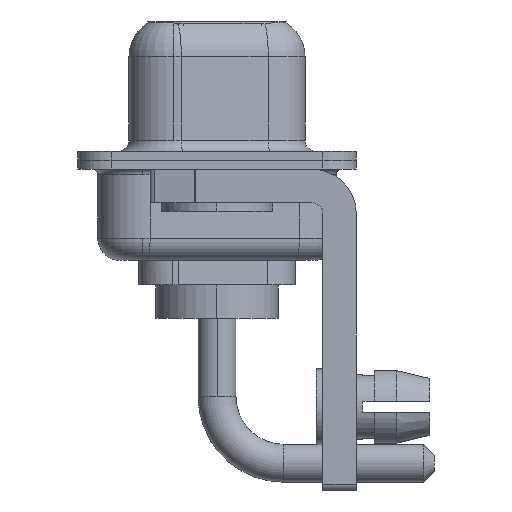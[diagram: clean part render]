
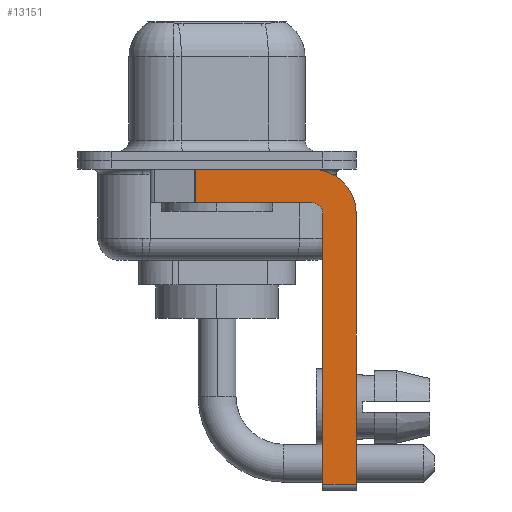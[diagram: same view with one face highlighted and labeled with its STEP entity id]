
A CAD part, left-side view. The second image highlights one B-rep face of the part: STEP entity #13151.
In plain terms, the highlighted planar face has unit normal (-1, 0, 0).
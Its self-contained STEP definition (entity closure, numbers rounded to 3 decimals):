
#184 = CARTESIAN_POINT ( 'NONE',  ( -2.9, 0.978, -0.4 ) ) ;
#433 = DIRECTION ( 'NONE',  ( 0., 0., -1. ) ) ;
#1268 = AXIS2_PLACEMENT_3D ( 'NONE', #6888, #1410, #1329 ) ;
#1329 = DIRECTION ( 'NONE',  ( 0., 0., -1. ) ) ;
#1383 = EDGE_CURVE ( 'NONE', #7160, #9571, #7773, .T. ) ;
#1410 = DIRECTION ( 'NONE',  ( 1., 0., 0. ) ) ;
#1455 = CARTESIAN_POINT ( 'NONE',  ( -2.9, -4.25, -1.9 ) ) ;
#1534 = ORIENTED_EDGE ( 'NONE', *, *, #4866, .F. ) ;
#2020 = ORIENTED_EDGE ( 'NONE', *, *, #12654, .F. ) ;
#2498 = VERTEX_POINT ( 'NONE', #10093 ) ;
#2610 = AXIS2_PLACEMENT_3D ( 'NONE', #8584, #3826, #433 ) ;
#2672 = DIRECTION ( 'NONE',  ( 0., 1., 0. ) ) ;
#2674 = ORIENTED_EDGE ( 'NONE', *, *, #14216, .F. ) ;
#2727 = VERTEX_POINT ( 'NONE', #4009 ) ;
#3349 = ORIENTED_EDGE ( 'NONE', *, *, #3689, .T. ) ;
#3541 = ORIENTED_EDGE ( 'NONE', *, *, #13024, .F. ) ;
#3608 = FACE_OUTER_BOUND ( 'NONE', #4203, .T. ) ;
#3689 = EDGE_CURVE ( 'NONE', #5356, #2498, #9668, .T. ) ;
#3821 = EDGE_CURVE ( 'NONE', #14453, #5346, #5415, .T. ) ;
#3826 = DIRECTION ( 'NONE',  ( 1., 0., 0. ) ) ;
#4009 = CARTESIAN_POINT ( 'NONE',  ( -2.9, -4.75, -2.4 ) ) ;
#4203 = EDGE_LOOP ( 'NONE', ( #1534, #3349, #2674, #3541, #2020, #13139, #8923, #10690 ) ) ;
#4320 = DIRECTION ( 'NONE',  ( 0., -1., 0. ) ) ;
#4866 = EDGE_CURVE ( 'NONE', #5356, #7160, #13252, .T. ) ;
#5322 = CARTESIAN_POINT ( 'NONE',  ( -2.9, -4.25, -0.4 ) ) ;
#5346 = VERTEX_POINT ( 'NONE', #10231 ) ;
#5356 = VERTEX_POINT ( 'NONE', #184 ) ;
#5415 = LINE ( 'NONE', #14397, #13348 ) ;
#5657 = DIRECTION ( 'NONE',  ( 0., -1., 0. ) ) ;
#5999 = PLANE ( 'NONE',  #1268 ) ;
#6609 = LINE ( 'NONE', #6741, #7544 ) ;
#6741 = CARTESIAN_POINT ( 'NONE',  ( -2.9, -6.25, -2.4 ) ) ;
#6888 = CARTESIAN_POINT ( 'NONE',  ( -2.9, -4.25, -2.4 ) ) ;
#7081 = VECTOR ( 'NONE', #11261, 1000. ) ;
#7160 = VERTEX_POINT ( 'NONE', #5322 ) ;
#7544 = VECTOR ( 'NONE', #7855, 1000. ) ;
#7579 = CARTESIAN_POINT ( 'NONE',  ( -2.9, -4.75, -14.55 ) ) ;
#7645 = CARTESIAN_POINT ( 'NONE',  ( -2.9, 3., -0.4 ) ) ;
#7679 = DIRECTION ( 'NONE',  ( 0., 0., -1. ) ) ;
#7773 = CIRCLE ( 'NONE', #2610, 2. ) ;
#7811 = LINE ( 'NONE', #12291, #7081 ) ;
#7855 = DIRECTION ( 'NONE',  ( 0., 0., -1. ) ) ;
#8394 = VECTOR ( 'NONE', #7679, 1000. ) ;
#8570 = CARTESIAN_POINT ( 'NONE',  ( -2.9, 0.978, -1.9 ) ) ;
#8584 = CARTESIAN_POINT ( 'NONE',  ( -2.9, -4.25, -2.4 ) ) ;
#8923 = ORIENTED_EDGE ( 'NONE', *, *, #11616, .F. ) ;
#9571 = VERTEX_POINT ( 'NONE', #14217 ) ;
#9575 = VECTOR ( 'NONE', #2672, 1000. ) ;
#9668 = LINE ( 'NONE', #8570, #8394 ) ;
#9917 = DIRECTION ( 'NONE',  ( -1., 0., 0. ) ) ;
#10093 = CARTESIAN_POINT ( 'NONE',  ( -2.9, 0.978, -1.9 ) ) ;
#10231 = CARTESIAN_POINT ( 'NONE',  ( -2.9, -6.25, -14.55 ) ) ;
#10372 = VERTEX_POINT ( 'NONE', #1455 ) ;
#10690 = ORIENTED_EDGE ( 'NONE', *, *, #1383, .F. ) ;
#11188 = VECTOR ( 'NONE', #5657, 1000. ) ;
#11261 = DIRECTION ( 'NONE',  ( 0., 0., 1. ) ) ;
#11328 = CIRCLE ( 'NONE', #12984, 0.5 ) ;
#11393 = LINE ( 'NONE', #13549, #9575 ) ;
#11616 = EDGE_CURVE ( 'NONE', #9571, #5346, #6609, .T. ) ;
#12291 = CARTESIAN_POINT ( 'NONE',  ( -2.9, -4.75, -14.8 ) ) ;
#12654 = EDGE_CURVE ( 'NONE', #14453, #2727, #7811, .T. ) ;
#12984 = AXIS2_PLACEMENT_3D ( 'NONE', #13392, #9917, #14429 ) ;
#13024 = EDGE_CURVE ( 'NONE', #2727, #10372, #11328, .T. ) ;
#13139 = ORIENTED_EDGE ( 'NONE', *, *, #3821, .T. ) ;
#13151 = ADVANCED_FACE ( 'NONE', ( #3608 ), #5999, .F. ) ;
#13252 = LINE ( 'NONE', #7645, #11188 ) ;
#13348 = VECTOR ( 'NONE', #4320, 1000. ) ;
#13392 = CARTESIAN_POINT ( 'NONE',  ( -2.9, -4.25, -2.4 ) ) ;
#13549 = CARTESIAN_POINT ( 'NONE',  ( -2.9, -4.25, -1.9 ) ) ;
#14216 = EDGE_CURVE ( 'NONE', #10372, #2498, #11393, .T. ) ;
#14217 = CARTESIAN_POINT ( 'NONE',  ( -2.9, -6.25, -2.4 ) ) ;
#14397 = CARTESIAN_POINT ( 'NONE',  ( -2.9, -4.25, -14.55 ) ) ;
#14429 = DIRECTION ( 'NONE',  ( 0., 0., 1. ) ) ;
#14453 = VERTEX_POINT ( 'NONE', #7579 ) ;
